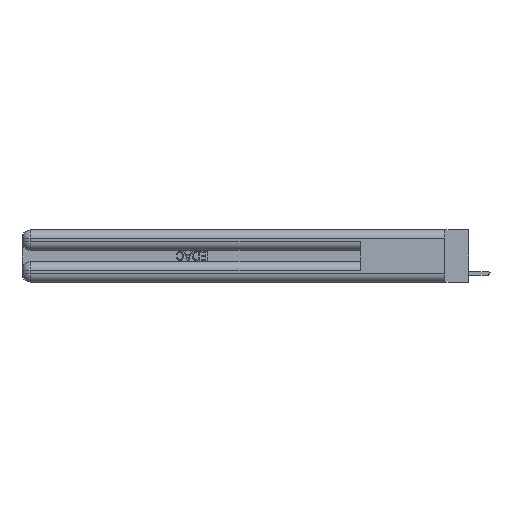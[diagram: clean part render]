
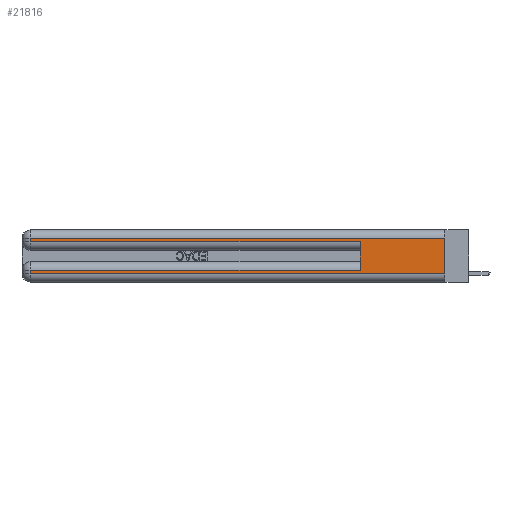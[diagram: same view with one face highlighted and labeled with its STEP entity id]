
A CAD part, left-side view. The second image highlights one B-rep face of the part: STEP entity #21816.
In plain terms, the highlighted planar face has unit normal (-1, 0, 0).
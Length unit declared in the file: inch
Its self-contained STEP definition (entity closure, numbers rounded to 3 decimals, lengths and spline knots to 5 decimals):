
#42 = VECTOR ( 'NONE', #8157, 39.37008 ) ;
#233 = VECTOR ( 'NONE', #21455, 39.37008 ) ;
#297 = PLANE ( 'NONE',  #5166 ) ;
#1246 = VECTOR ( 'NONE', #22033, 39.37008 ) ;
#1666 = DIRECTION ( 'NONE',  ( 0., 0., -1. ) ) ;
#1828 = EDGE_CURVE ( 'NONE', #12920, #20538, #10500, .T. ) ;
#3136 = DIRECTION ( 'NONE',  ( 0., 0., -1. ) ) ;
#3265 = VECTOR ( 'NONE', #16808, 39.37008 ) ;
#3673 = EDGE_CURVE ( 'NONE', #14492, #24007, #22287, .T. ) ;
#5166 = AXIS2_PLACEMENT_3D ( 'NONE', #15879, #24879, #17869 ) ;
#5505 = LINE ( 'NONE', #6057, #22227 ) ;
#5637 = VECTOR ( 'NONE', #3136, 39.37008 ) ;
#6057 = CARTESIAN_POINT ( 'NONE',  ( 0., 2.94, 0.37 ) ) ;
#6088 = EDGE_LOOP ( 'NONE', ( #28995, #24399, #7481, #21980, #18589, #17453, #17408, #10274 ) ) ;
#6256 = CARTESIAN_POINT ( 'NONE',  ( 0., 0., 0.06 ) ) ;
#7481 = ORIENTED_EDGE ( 'NONE', *, *, #10664, .T. ) ;
#7712 = VERTEX_POINT ( 'NONE', #18224 ) ;
#8157 = DIRECTION ( 'NONE',  ( 0., 1., 0. ) ) ;
#9429 = VERTEX_POINT ( 'NONE', #14357 ) ;
#9671 = DIRECTION ( 'NONE',  ( 0., 0., 1. ) ) ;
#10274 = ORIENTED_EDGE ( 'NONE', *, *, #21657, .T. ) ;
#10283 = CARTESIAN_POINT ( 'NONE',  ( 0., 0.6, 0.285 ) ) ;
#10500 = LINE ( 'NONE', #11966, #5637 ) ;
#10664 = EDGE_CURVE ( 'NONE', #10694, #14492, #5505, .T. ) ;
#10694 = VERTEX_POINT ( 'NONE', #10703 ) ;
#10703 = CARTESIAN_POINT ( 'NONE',  ( 0., 2.94, 0.31 ) ) ;
#11710 = VERTEX_POINT ( 'NONE', #22357 ) ;
#11966 = CARTESIAN_POINT ( 'NONE',  ( 0., 2.94, 0.37 ) ) ;
#12441 = LINE ( 'NONE', #28553, #233 ) ;
#12621 = LINE ( 'NONE', #20826, #13283 ) ;
#12920 = VERTEX_POINT ( 'NONE', #19872 ) ;
#13283 = VECTOR ( 'NONE', #9671, 39.37008 ) ;
#14187 = EDGE_CURVE ( 'NONE', #11710, #12920, #26645, .T. ) ;
#14357 = CARTESIAN_POINT ( 'NONE',  ( 0., 0., 0.06 ) ) ;
#14413 = EDGE_CURVE ( 'NONE', #11710, #24007, #12621, .T. ) ;
#14492 = VERTEX_POINT ( 'NONE', #18782 ) ;
#15298 = CARTESIAN_POINT ( 'NONE',  ( 0., 2.94, 0.06 ) ) ;
#15879 = CARTESIAN_POINT ( 'NONE',  ( 0., 0., 0.37 ) ) ;
#15987 = CARTESIAN_POINT ( 'NONE',  ( 0., 0., 0.285 ) ) ;
#16808 = DIRECTION ( 'NONE',  ( 0., 1., 0. ) ) ;
#17014 = CARTESIAN_POINT ( 'NONE',  ( 0., 0., 0.31 ) ) ;
#17078 = VECTOR ( 'NONE', #20408, 39.37008 ) ;
#17408 = ORIENTED_EDGE ( 'NONE', *, *, #1828, .T. ) ;
#17453 = ORIENTED_EDGE ( 'NONE', *, *, #14187, .T. ) ;
#17869 = DIRECTION ( 'NONE',  ( 0., 0., -1. ) ) ;
#18224 = CARTESIAN_POINT ( 'NONE',  ( 0., 0., 0.31 ) ) ;
#18589 = ORIENTED_EDGE ( 'NONE', *, *, #14413, .F. ) ;
#18782 = CARTESIAN_POINT ( 'NONE',  ( 0., 2.94, 0.285 ) ) ;
#19289 = CARTESIAN_POINT ( 'NONE',  ( 0., 0., 0.085 ) ) ;
#19872 = CARTESIAN_POINT ( 'NONE',  ( 0., 2.94, 0.085 ) ) ;
#20375 = EDGE_CURVE ( 'NONE', #7712, #10694, #26666, .T. ) ;
#20408 = DIRECTION ( 'NONE',  ( 0., -1., 0. ) ) ;
#20538 = VERTEX_POINT ( 'NONE', #15298 ) ;
#20826 = CARTESIAN_POINT ( 'NONE',  ( 0., 0.6, 0.145 ) ) ;
#21112 = FACE_OUTER_BOUND ( 'NONE', #6088, .T. ) ;
#21455 = DIRECTION ( 'NONE',  ( 0., 0., -1. ) ) ;
#21464 = LINE ( 'NONE', #6256, #1246 ) ;
#21657 = EDGE_CURVE ( 'NONE', #20538, #9429, #21464, .T. ) ;
#21816 = ADVANCED_FACE ( 'NONE', ( #21112 ), #297, .F. ) ;
#21980 = ORIENTED_EDGE ( 'NONE', *, *, #3673, .T. ) ;
#22033 = DIRECTION ( 'NONE',  ( 0., -1., 0. ) ) ;
#22227 = VECTOR ( 'NONE', #1666, 39.37008 ) ;
#22287 = LINE ( 'NONE', #15987, #17078 ) ;
#22357 = CARTESIAN_POINT ( 'NONE',  ( 0., 0.6, 0.085 ) ) ;
#24007 = VERTEX_POINT ( 'NONE', #10283 ) ;
#24399 = ORIENTED_EDGE ( 'NONE', *, *, #20375, .T. ) ;
#24879 = DIRECTION ( 'NONE',  ( 1., 0., 0. ) ) ;
#26645 = LINE ( 'NONE', #19289, #42 ) ;
#26666 = LINE ( 'NONE', #17014, #3265 ) ;
#26988 = EDGE_CURVE ( 'NONE', #7712, #9429, #12441, .T. ) ;
#28553 = CARTESIAN_POINT ( 'NONE',  ( 0., 0., 0.37 ) ) ;
#28995 = ORIENTED_EDGE ( 'NONE', *, *, #26988, .F. ) ;
